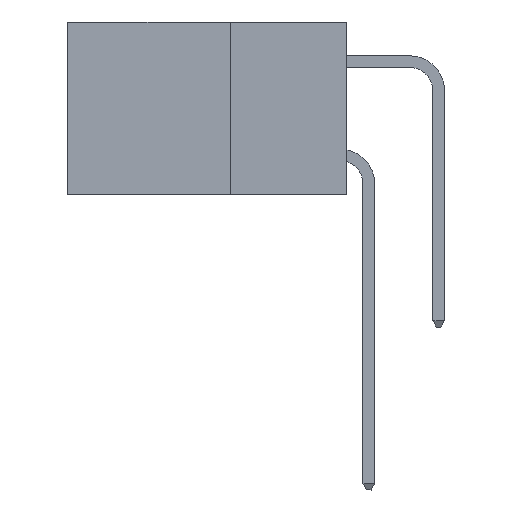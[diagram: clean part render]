
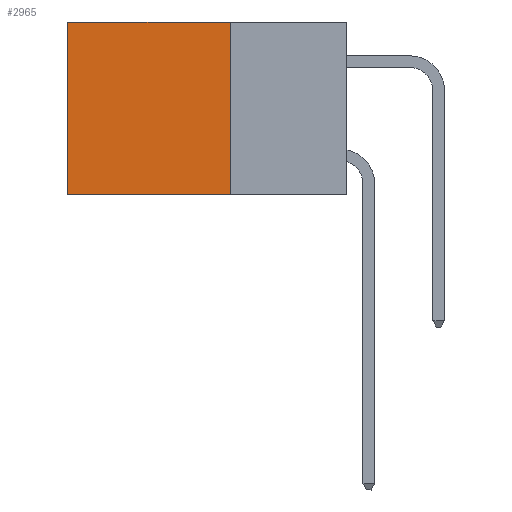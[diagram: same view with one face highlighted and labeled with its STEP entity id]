
A CAD part, left-side view. The second image highlights one B-rep face of the part: STEP entity #2965.
In plain terms, the highlighted planar face has unit normal (-1, 0, 0).
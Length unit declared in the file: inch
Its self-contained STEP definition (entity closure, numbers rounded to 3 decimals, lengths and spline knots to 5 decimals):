
#311 = VECTOR ( 'NONE', #8676, 39.37008 ) ;
#617 = AXIS2_PLACEMENT_3D ( 'NONE', #12499, #6628, #13522 ) ;
#623 = LINE ( 'NONE', #7702, #4949 ) ;
#1316 = VERTEX_POINT ( 'NONE', #8668 ) ;
#1354 = DIRECTION ( 'NONE',  ( 0., 0., -1. ) ) ;
#1913 = EDGE_CURVE ( 'NONE', #1316, #5687, #623, .T. ) ;
#2385 = FACE_OUTER_BOUND ( 'NONE', #11099, .T. ) ;
#2965 = ADVANCED_FACE ( 'NONE', ( #2385 ), #3775, .F. ) ;
#2969 = CARTESIAN_POINT ( 'NONE',  ( 0.2875, 0.6, 0. ) ) ;
#3775 = PLANE ( 'NONE',  #617 ) ;
#3911 = DIRECTION ( 'NONE',  ( 0., 1., 0. ) ) ;
#4715 = LINE ( 'NONE', #2969, #311 ) ;
#4949 = VECTOR ( 'NONE', #7520, 39.37008 ) ;
#4965 = VECTOR ( 'NONE', #1354, 39.37008 ) ;
#5687 = VERTEX_POINT ( 'NONE', #13873 ) ;
#6033 = CARTESIAN_POINT ( 'NONE',  ( 0.2875, 0.25, 0. ) ) ;
#6524 = ORIENTED_EDGE ( 'NONE', *, *, #16240, .T. ) ;
#6628 = DIRECTION ( 'NONE',  ( 1., 0., 0. ) ) ;
#6682 = VECTOR ( 'NONE', #3911, 39.37008 ) ;
#6792 = LINE ( 'NONE', #15332, #4965 ) ;
#7520 = DIRECTION ( 'NONE',  ( 0., 1., 0. ) ) ;
#7702 = CARTESIAN_POINT ( 'NONE',  ( 0.2875, 0.25, -0.37 ) ) ;
#8668 = CARTESIAN_POINT ( 'NONE',  ( 0.2875, 0.25, -0.37 ) ) ;
#8676 = DIRECTION ( 'NONE',  ( 0., 0., -1. ) ) ;
#9344 = VERTEX_POINT ( 'NONE', #6033 ) ;
#9838 = ORIENTED_EDGE ( 'NONE', *, *, #12280, .T. ) ;
#11099 = EDGE_LOOP ( 'NONE', ( #6524, #15388, #12433, #9838 ) ) ;
#12280 = EDGE_CURVE ( 'NONE', #9344, #13173, #15482, .T. ) ;
#12314 = CARTESIAN_POINT ( 'NONE',  ( 0.2875, 0.6, 0. ) ) ;
#12433 = ORIENTED_EDGE ( 'NONE', *, *, #13929, .F. ) ;
#12499 = CARTESIAN_POINT ( 'NONE',  ( 0.2875, 0.25, 0. ) ) ;
#13173 = VERTEX_POINT ( 'NONE', #12314 ) ;
#13522 = DIRECTION ( 'NONE',  ( 0., 0., -1. ) ) ;
#13841 = CARTESIAN_POINT ( 'NONE',  ( 0.2875, 0.25, 0. ) ) ;
#13873 = CARTESIAN_POINT ( 'NONE',  ( 0.2875, 0.6, -0.37 ) ) ;
#13929 = EDGE_CURVE ( 'NONE', #9344, #1316, #6792, .T. ) ;
#15332 = CARTESIAN_POINT ( 'NONE',  ( 0.2875, 0.25, 0. ) ) ;
#15388 = ORIENTED_EDGE ( 'NONE', *, *, #1913, .F. ) ;
#15482 = LINE ( 'NONE', #13841, #6682 ) ;
#16240 = EDGE_CURVE ( 'NONE', #13173, #5687, #4715, .T. ) ;
